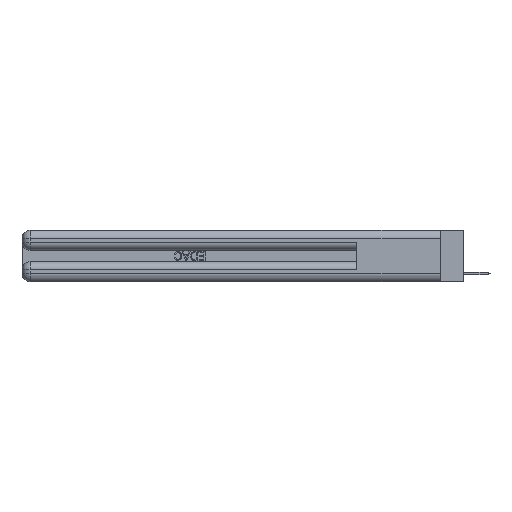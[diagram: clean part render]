
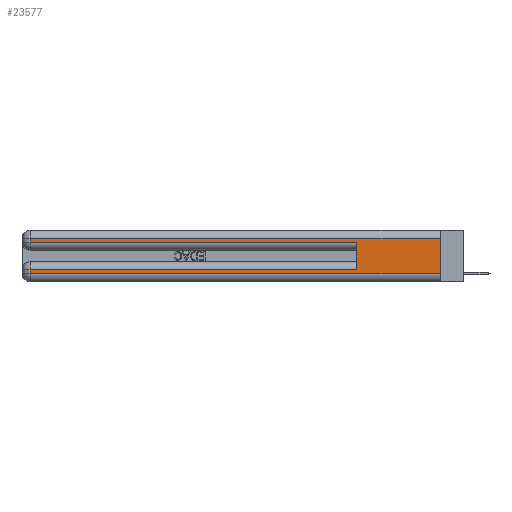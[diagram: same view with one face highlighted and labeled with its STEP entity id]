
A CAD part, left-side view. The second image highlights one B-rep face of the part: STEP entity #23577.
In plain terms, the highlighted planar face has unit normal (-1, 0, 0).
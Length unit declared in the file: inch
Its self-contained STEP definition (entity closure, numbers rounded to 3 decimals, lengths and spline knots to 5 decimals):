
#92 = ORIENTED_EDGE ( 'NONE', *, *, #14852, .T. ) ;
#199 = LINE ( 'NONE', #7309, #17625 ) ;
#1969 = VECTOR ( 'NONE', #7294, 39.37008 ) ;
#2598 = AXIS2_PLACEMENT_3D ( 'NONE', #19673, #2944, #2808 ) ;
#2662 = VECTOR ( 'NONE', #20860, 39.37008 ) ;
#2808 = DIRECTION ( 'NONE',  ( 0., 0., -1. ) ) ;
#2944 = DIRECTION ( 'NONE',  ( 1., 0., 0. ) ) ;
#2979 = CARTESIAN_POINT ( 'NONE',  ( 0., 0., 0.06 ) ) ;
#2989 = DIRECTION ( 'NONE',  ( 0., 0., 1. ) ) ;
#3594 = DIRECTION ( 'NONE',  ( 0., 1., 0. ) ) ;
#3639 = ORIENTED_EDGE ( 'NONE', *, *, #23336, .T. ) ;
#4079 = VECTOR ( 'NONE', #2989, 39.37008 ) ;
#4506 = FACE_OUTER_BOUND ( 'NONE', #4737, .T. ) ;
#4628 = DIRECTION ( 'NONE',  ( 0., -1., 0. ) ) ;
#4731 = CARTESIAN_POINT ( 'NONE',  ( 0., 0., 0.31 ) ) ;
#4737 = EDGE_LOOP ( 'NONE', ( #27544, #92, #11881, #16104, #15753, #19954, #3639, #26184 ) ) ;
#5139 = LINE ( 'NONE', #5417, #4079 ) ;
#5153 = VERTEX_POINT ( 'NONE', #22319 ) ;
#5225 = CARTESIAN_POINT ( 'NONE',  ( 0., 0., 0.06 ) ) ;
#5320 = LINE ( 'NONE', #11839, #1969 ) ;
#5417 = CARTESIAN_POINT ( 'NONE',  ( 0., 0.6, 0.145 ) ) ;
#5513 = DIRECTION ( 'NONE',  ( 0., -1., 0. ) ) ;
#5586 = EDGE_CURVE ( 'NONE', #18932, #12018, #5139, .T. ) ;
#5774 = LINE ( 'NONE', #5225, #13310 ) ;
#5792 = VECTOR ( 'NONE', #20829, 39.37008 ) ;
#6439 = VERTEX_POINT ( 'NONE', #12093 ) ;
#6721 = CARTESIAN_POINT ( 'NONE',  ( 0., 0.6, 0.285 ) ) ;
#6740 = VERTEX_POINT ( 'NONE', #11507 ) ;
#7294 = DIRECTION ( 'NONE',  ( 0., 1., 0. ) ) ;
#7309 = CARTESIAN_POINT ( 'NONE',  ( 0., 0., 0.285 ) ) ;
#7810 = LINE ( 'NONE', #16462, #2662 ) ;
#8046 = CARTESIAN_POINT ( 'NONE',  ( 0., 2.94, 0.37 ) ) ;
#8301 = CARTESIAN_POINT ( 'NONE',  ( 0., 0.6, 0.085 ) ) ;
#11507 = CARTESIAN_POINT ( 'NONE',  ( 0., 2.94, 0.31 ) ) ;
#11839 = CARTESIAN_POINT ( 'NONE',  ( 0., 0., 0.31 ) ) ;
#11881 = ORIENTED_EDGE ( 'NONE', *, *, #26746, .T. ) ;
#12018 = VERTEX_POINT ( 'NONE', #6721 ) ;
#12093 = CARTESIAN_POINT ( 'NONE',  ( 0., 2.94, 0.285 ) ) ;
#12183 = LINE ( 'NONE', #8046, #5792 ) ;
#13310 = VECTOR ( 'NONE', #5513, 39.37008 ) ;
#13680 = CARTESIAN_POINT ( 'NONE',  ( 0., 2.94, 0.085 ) ) ;
#14140 = LINE ( 'NONE', #26913, #22835 ) ;
#14506 = CARTESIAN_POINT ( 'NONE',  ( 0., 0., 0.085 ) ) ;
#14852 = EDGE_CURVE ( 'NONE', #19526, #6740, #5320, .T. ) ;
#15409 = PLANE ( 'NONE',  #2598 ) ;
#15753 = ORIENTED_EDGE ( 'NONE', *, *, #5586, .F. ) ;
#16104 = ORIENTED_EDGE ( 'NONE', *, *, #27918, .T. ) ;
#16462 = CARTESIAN_POINT ( 'NONE',  ( 0., 2.94, 0.37 ) ) ;
#17442 = EDGE_CURVE ( 'NONE', #5153, #23229, #5774, .T. ) ;
#17477 = EDGE_CURVE ( 'NONE', #19526, #23229, #14140, .T. ) ;
#17625 = VECTOR ( 'NONE', #4628, 39.37008 ) ;
#18932 = VERTEX_POINT ( 'NONE', #8301 ) ;
#19039 = LINE ( 'NONE', #14506, #26617 ) ;
#19526 = VERTEX_POINT ( 'NONE', #4731 ) ;
#19673 = CARTESIAN_POINT ( 'NONE',  ( 0., 0., 0.37 ) ) ;
#19954 = ORIENTED_EDGE ( 'NONE', *, *, #23135, .T. ) ;
#20829 = DIRECTION ( 'NONE',  ( 0., 0., -1. ) ) ;
#20860 = DIRECTION ( 'NONE',  ( 0., 0., -1. ) ) ;
#22319 = CARTESIAN_POINT ( 'NONE',  ( 0., 2.94, 0.06 ) ) ;
#22648 = DIRECTION ( 'NONE',  ( 0., 0., -1. ) ) ;
#22835 = VECTOR ( 'NONE', #22648, 39.37008 ) ;
#23135 = EDGE_CURVE ( 'NONE', #18932, #25049, #19039, .T. ) ;
#23229 = VERTEX_POINT ( 'NONE', #2979 ) ;
#23336 = EDGE_CURVE ( 'NONE', #25049, #5153, #12183, .T. ) ;
#23577 = ADVANCED_FACE ( 'NONE', ( #4506 ), #15409, .F. ) ;
#25049 = VERTEX_POINT ( 'NONE', #13680 ) ;
#26184 = ORIENTED_EDGE ( 'NONE', *, *, #17442, .T. ) ;
#26617 = VECTOR ( 'NONE', #3594, 39.37008 ) ;
#26746 = EDGE_CURVE ( 'NONE', #6740, #6439, #7810, .T. ) ;
#26913 = CARTESIAN_POINT ( 'NONE',  ( 0., 0., 0.37 ) ) ;
#27544 = ORIENTED_EDGE ( 'NONE', *, *, #17477, .F. ) ;
#27918 = EDGE_CURVE ( 'NONE', #6439, #12018, #199, .T. ) ;
